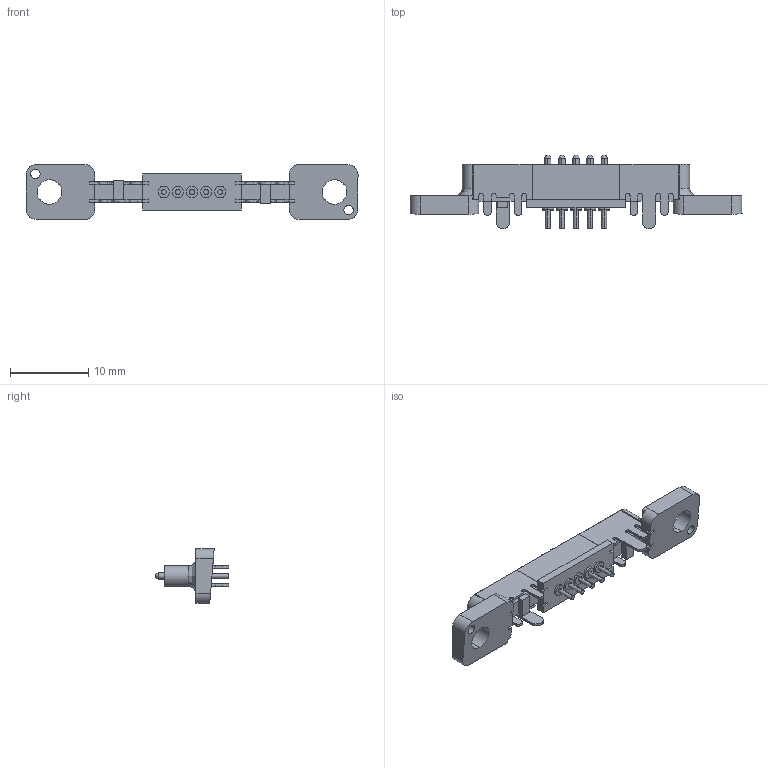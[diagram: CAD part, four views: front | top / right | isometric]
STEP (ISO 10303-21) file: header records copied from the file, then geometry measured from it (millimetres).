
FILE_DESCRIPTION (( 'STEP AP214' ), '1' );
FILE_NAME ('685F05C4211113Q.STEP', '2023-04-25T18:41:18', ( '' ), ( '' ), 'SwSTEP 2.0', 'SolidWorks 2020', '' );
FILE_SCHEMA (( 'AUTOMOTIVE_DESIGN' ));
Length unit declared in the file: millimetre
Products named in the file (1): 685F05C4211113Q
Bounding box: 42.4 x 9.4 x 7 mm (x, y, z)
Volume: 609.9 mm3; surface area: 1606.7 mm2
Topology: 5 solids, 5 shells, 365 faces, 944 edges, 588 vertices
Faces by surface type: plane 208, cylinder 128, bspline 27, cone 2
Entity records: 15275 total; most frequent: CARTESIAN_POINT 2436, ORIENTED_EDGE 1836, DIRECTION 1825, EDGE_CURVE 918, VECTOR 639, LINE 639, AXIS2_PLACEMENT_3D 593, VERTEX_POINT 588
